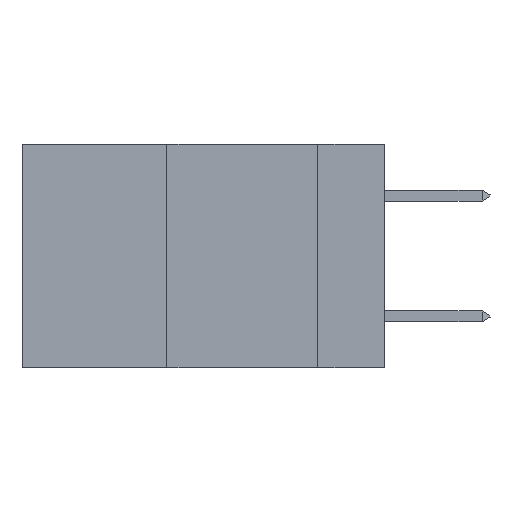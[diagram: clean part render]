
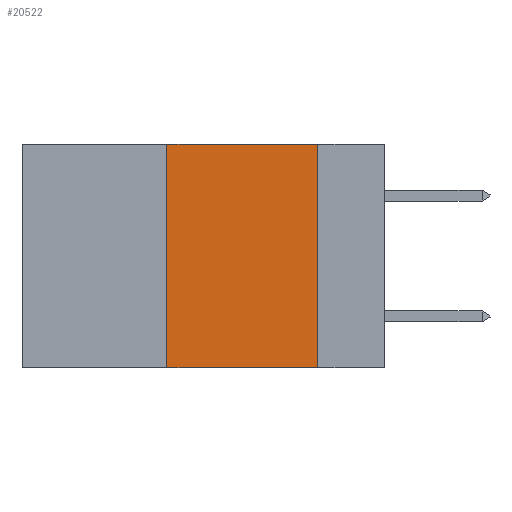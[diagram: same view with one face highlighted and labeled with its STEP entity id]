
A CAD part, left-side view. The second image highlights one B-rep face of the part: STEP entity #20522.
In plain terms, the highlighted planar face has unit normal (-1, 0, 0).
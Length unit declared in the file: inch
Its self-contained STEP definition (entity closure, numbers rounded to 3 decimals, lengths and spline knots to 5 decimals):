
#735 = EDGE_LOOP ( 'NONE', ( #27520, #29770, #2973, #39238 ) ) ;
#2973 = ORIENTED_EDGE ( 'NONE', *, *, #12046, .F. ) ;
#3170 = CARTESIAN_POINT ( 'NONE',  ( 0., 0.6, 0. ) ) ;
#3486 = DIRECTION ( 'NONE',  ( 0., 0., -1. ) ) ;
#4462 = VECTOR ( 'NONE', #31181, 39.37008 ) ;
#5839 = EDGE_CURVE ( 'NONE', #8101, #20350, #33144, .T. ) ;
#6746 = VERTEX_POINT ( 'NONE', #14549 ) ;
#8101 = VERTEX_POINT ( 'NONE', #19120 ) ;
#9326 = AXIS2_PLACEMENT_3D ( 'NONE', #13492, #27089, #3486 ) ;
#9479 = EDGE_CURVE ( 'NONE', #20350, #34323, #22995, .T. ) ;
#11981 = LINE ( 'NONE', #12257, #18477 ) ;
#12046 = EDGE_CURVE ( 'NONE', #6746, #8101, #11981, .T. ) ;
#12257 = CARTESIAN_POINT ( 'NONE',  ( 0., 0.36, 0. ) ) ;
#13492 = CARTESIAN_POINT ( 'NONE',  ( 0., 0.6, 0. ) ) ;
#14549 = CARTESIAN_POINT ( 'NONE',  ( 0., 0.36, -0.37 ) ) ;
#16326 = CARTESIAN_POINT ( 'NONE',  ( 0., 0.11, 0. ) ) ;
#18477 = VECTOR ( 'NONE', #33130, 39.37008 ) ;
#19120 = CARTESIAN_POINT ( 'NONE',  ( 0., 0.36, 0. ) ) ;
#19606 = FACE_OUTER_BOUND ( 'NONE', #735, .T. ) ;
#19699 = PLANE ( 'NONE',  #9326 ) ;
#20350 = VERTEX_POINT ( 'NONE', #22431 ) ;
#20522 = ADVANCED_FACE ( 'NONE', ( #19606 ), #19699, .F. ) ;
#21910 = VECTOR ( 'NONE', #40817, 39.37008 ) ;
#22431 = CARTESIAN_POINT ( 'NONE',  ( 0., 0.11, 0. ) ) ;
#22995 = LINE ( 'NONE', #16326, #21910 ) ;
#25749 = LINE ( 'NONE', #34840, #33898 ) ;
#25832 = EDGE_CURVE ( 'NONE', #6746, #34323, #25749, .T. ) ;
#27089 = DIRECTION ( 'NONE',  ( 1., 0., 0. ) ) ;
#27520 = ORIENTED_EDGE ( 'NONE', *, *, #9479, .F. ) ;
#29770 = ORIENTED_EDGE ( 'NONE', *, *, #5839, .F. ) ;
#31181 = DIRECTION ( 'NONE',  ( 0., -1., 0. ) ) ;
#33130 = DIRECTION ( 'NONE',  ( 0., 0., 1. ) ) ;
#33144 = LINE ( 'NONE', #3170, #4462 ) ;
#33898 = VECTOR ( 'NONE', #38317, 39.37008 ) ;
#34323 = VERTEX_POINT ( 'NONE', #34799 ) ;
#34799 = CARTESIAN_POINT ( 'NONE',  ( 0., 0.11, -0.37 ) ) ;
#34840 = CARTESIAN_POINT ( 'NONE',  ( 0., 0.6, -0.37 ) ) ;
#38317 = DIRECTION ( 'NONE',  ( 0., -1., 0. ) ) ;
#39238 = ORIENTED_EDGE ( 'NONE', *, *, #25832, .T. ) ;
#40817 = DIRECTION ( 'NONE',  ( 0., 0., -1. ) ) ;
